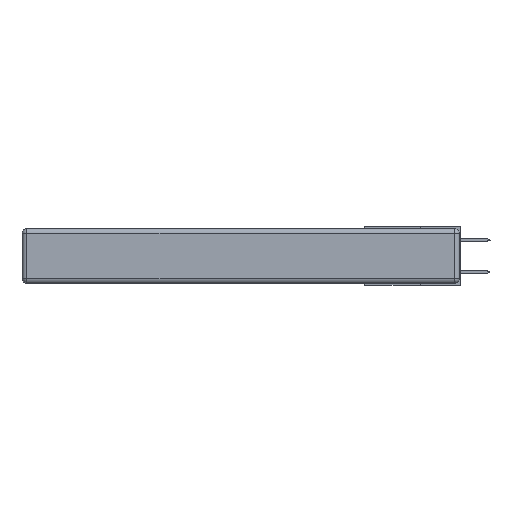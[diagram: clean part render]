
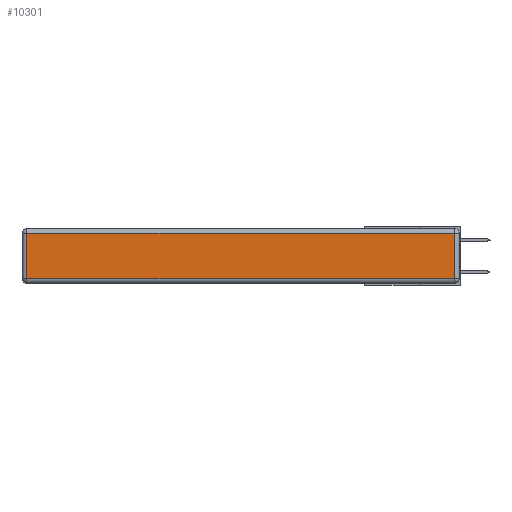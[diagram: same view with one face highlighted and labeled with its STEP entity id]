
A CAD part, left-side view. The second image highlights one B-rep face of the part: STEP entity #10301.
In plain terms, the highlighted planar face has unit normal (-1, 0, 0).
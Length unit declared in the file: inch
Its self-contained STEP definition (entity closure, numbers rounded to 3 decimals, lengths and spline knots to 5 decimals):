
#73 = LINE ( 'NONE', #2310, #4349 ) ;
#1058 = DIRECTION ( 'NONE',  ( 0., 1., 0. ) ) ;
#1586 = ORIENTED_EDGE ( 'NONE', *, *, #9887, .T. ) ;
#2098 = EDGE_CURVE ( 'NONE', #4347, #7375, #10469, .T. ) ;
#2310 = CARTESIAN_POINT ( 'NONE',  ( 0., 2.72, -0.343 ) ) ;
#2468 = DIRECTION ( 'NONE',  ( 0., 0., 1. ) ) ;
#2708 = CARTESIAN_POINT ( 'NONE',  ( 0., 0.03, -0.343 ) ) ;
#2897 = CARTESIAN_POINT ( 'NONE',  ( 0., 2.75, -0.03 ) ) ;
#3144 = LINE ( 'NONE', #7942, #9465 ) ;
#3188 = DIRECTION ( 'NONE',  ( 0., -1., 0. ) ) ;
#3246 = CARTESIAN_POINT ( 'NONE',  ( 0., 0., -0.343 ) ) ;
#3728 = VERTEX_POINT ( 'NONE', #5694 ) ;
#3944 = CARTESIAN_POINT ( 'NONE',  ( 0., 0.03, -0.03 ) ) ;
#4347 = VERTEX_POINT ( 'NONE', #3944 ) ;
#4349 = VECTOR ( 'NONE', #8826, 39.37008 ) ;
#5066 = VERTEX_POINT ( 'NONE', #7232 ) ;
#5332 = ORIENTED_EDGE ( 'NONE', *, *, #6564, .T. ) ;
#5694 = CARTESIAN_POINT ( 'NONE',  ( 0., 0.03, -0.313 ) ) ;
#6159 = CARTESIAN_POINT ( 'NONE',  ( 0., 2.72, -0.03 ) ) ;
#6564 = EDGE_CURVE ( 'NONE', #7375, #5066, #73, .T. ) ;
#7011 = ORIENTED_EDGE ( 'NONE', *, *, #8084, .T. ) ;
#7232 = CARTESIAN_POINT ( 'NONE',  ( 0., 2.72, -0.313 ) ) ;
#7375 = VERTEX_POINT ( 'NONE', #6159 ) ;
#7942 = CARTESIAN_POINT ( 'NONE',  ( 0., 0., -0.313 ) ) ;
#8084 = EDGE_CURVE ( 'NONE', #3728, #4347, #11121, .T. ) ;
#8113 = DIRECTION ( 'NONE',  ( -1., 0., 0. ) ) ;
#8299 = EDGE_LOOP ( 'NONE', ( #1586, #7011, #9287, #5332 ) ) ;
#8826 = DIRECTION ( 'NONE',  ( 0., 0., -1. ) ) ;
#8867 = PLANE ( 'NONE',  #9710 ) ;
#9147 = DIRECTION ( 'NONE',  ( 0., 0., 1. ) ) ;
#9287 = ORIENTED_EDGE ( 'NONE', *, *, #2098, .T. ) ;
#9344 = VECTOR ( 'NONE', #9147, 39.37008 ) ;
#9465 = VECTOR ( 'NONE', #3188, 39.37008 ) ;
#9710 = AXIS2_PLACEMENT_3D ( 'NONE', #3246, #8113, #2468 ) ;
#9887 = EDGE_CURVE ( 'NONE', #5066, #3728, #3144, .T. ) ;
#10131 = FACE_OUTER_BOUND ( 'NONE', #8299, .T. ) ;
#10301 = ADVANCED_FACE ( 'NONE', ( #10131 ), #8867, .T. ) ;
#10469 = LINE ( 'NONE', #2897, #11643 ) ;
#11121 = LINE ( 'NONE', #2708, #9344 ) ;
#11643 = VECTOR ( 'NONE', #1058, 39.37008 ) ;
